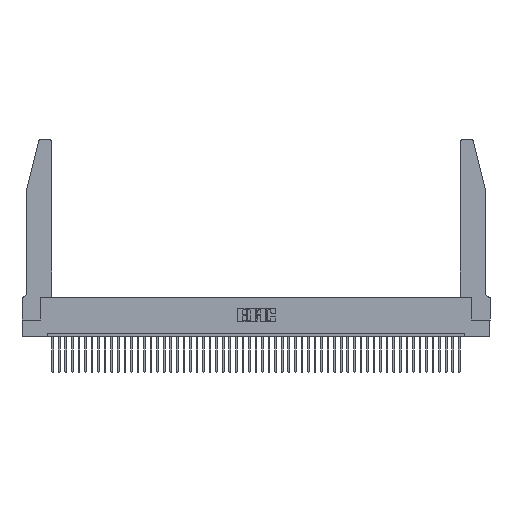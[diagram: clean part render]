
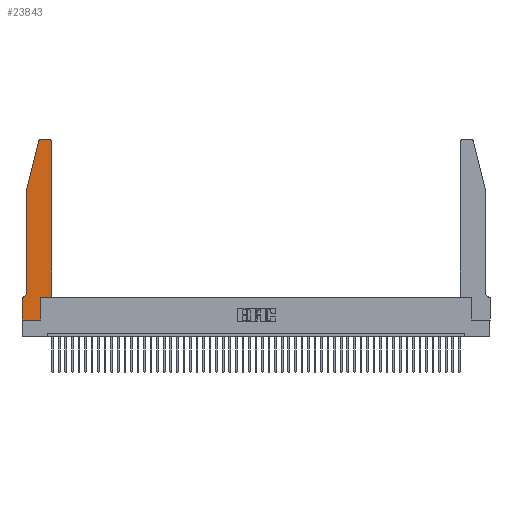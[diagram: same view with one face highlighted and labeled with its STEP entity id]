
A CAD part, top view. The second image highlights one B-rep face of the part: STEP entity #23843.
In plain terms, the highlighted planar face has unit normal (0, 0, 1).
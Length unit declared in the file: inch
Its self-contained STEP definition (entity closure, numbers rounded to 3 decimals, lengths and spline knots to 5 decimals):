
#1245 = DIRECTION ( 'NONE',  ( 1., 0., 0. ) ) ;
#1791 = LINE ( 'NONE', #37904, #36975 ) ;
#1830 = CARTESIAN_POINT ( 'NONE',  ( 0.4505, 0.35, 0.37 ) ) ;
#2072 = ORIENTED_EDGE ( 'NONE', *, *, #17591, .T. ) ;
#2438 = VERTEX_POINT ( 'NONE', #41297 ) ;
#2850 = AXIS2_PLACEMENT_3D ( 'NONE', #13372, #17579, #48704 ) ;
#2998 = EDGE_CURVE ( 'NONE', #13315, #28401, #1791, .T. ) ;
#3401 = LINE ( 'NONE', #48286, #9929 ) ;
#4139 = ORIENTED_EDGE ( 'NONE', *, *, #20110, .T. ) ;
#4287 = EDGE_CURVE ( 'NONE', #31102, #2438, #5827, .T. ) ;
#4763 = EDGE_CURVE ( 'NONE', #47648, #45885, #19547, .T. ) ;
#5475 = CARTESIAN_POINT ( 'NONE',  ( 0.2605, 2.75, 0.37 ) ) ;
#5827 = LINE ( 'NONE', #14766, #17216 ) ;
#6153 = LINE ( 'NONE', #5475, #27068 ) ;
#6427 = DIRECTION ( 'NONE',  ( 0., 1., 0. ) ) ;
#6703 = DIRECTION ( 'NONE',  ( 0., -1., 0. ) ) ;
#6869 = DIRECTION ( 'NONE',  ( 1., 0., 0. ) ) ;
#7040 = DIRECTION ( 'NONE',  ( 0., 0., 1. ) ) ;
#8311 = LINE ( 'NONE', #36016, #35166 ) ;
#8898 = DIRECTION ( 'NONE',  ( 0., 0., 1. ) ) ;
#9929 = VECTOR ( 'NONE', #6427, 39.37008 ) ;
#10194 = EDGE_CURVE ( 'NONE', #40480, #47648, #6153, .T. ) ;
#10562 = PLANE ( 'NONE',  #42308 ) ;
#11582 = AXIS2_PLACEMENT_3D ( 'NONE', #20313, #8898, #1245 ) ;
#11965 = VECTOR ( 'NONE', #31570, 39.37008 ) ;
#13315 = VERTEX_POINT ( 'NONE', #31732 ) ;
#13372 = CARTESIAN_POINT ( 'NONE',  ( 0.284, 2.72, 0.37 ) ) ;
#13621 = LINE ( 'NONE', #28148, #42801 ) ;
#13745 = CARTESIAN_POINT ( 'NONE',  ( 0.0755, 0.42, 0.37 ) ) ;
#14268 = CARTESIAN_POINT ( 'NONE',  ( 0.0055, 0.42, 0.37 ) ) ;
#14766 = CARTESIAN_POINT ( 'NONE',  ( 0., 0., 0.37 ) ) ;
#15083 = CARTESIAN_POINT ( 'NONE',  ( 0.4205, 2.75, 0.37 ) ) ;
#15116 = ORIENTED_EDGE ( 'NONE', *, *, #10194, .T. ) ;
#16860 = DIRECTION ( 'NONE',  ( 1., 0., 0. ) ) ;
#16972 = VERTEX_POINT ( 'NONE', #39715 ) ;
#17179 = ORIENTED_EDGE ( 'NONE', *, *, #45188, .T. ) ;
#17216 = VECTOR ( 'NONE', #26597, 39.37008 ) ;
#17579 = DIRECTION ( 'NONE',  ( 0., 0., 1. ) ) ;
#17591 = EDGE_CURVE ( 'NONE', #39319, #31102, #13621, .T. ) ;
#17788 = VECTOR ( 'NONE', #25382, 39.37008 ) ;
#18202 = FACE_OUTER_BOUND ( 'NONE', #48448, .T. ) ;
#19417 = ORIENTED_EDGE ( 'NONE', *, *, #29807, .T. ) ;
#19547 = CIRCLE ( 'NONE', #2850, 0.03 ) ;
#20110 = EDGE_CURVE ( 'NONE', #39949, #40480, #20575, .T. ) ;
#20198 = ORIENTED_EDGE ( 'NONE', *, *, #43814, .T. ) ;
#20313 = CARTESIAN_POINT ( 'NONE',  ( 0.4205, 2.72, 0.37 ) ) ;
#20343 = CARTESIAN_POINT ( 'NONE',  ( 0.284, 2.75, 0.37 ) ) ;
#20352 = LINE ( 'NONE', #48483, #25751 ) ;
#20575 = CIRCLE ( 'NONE', #11582, 0.03 ) ;
#21649 = DIRECTION ( 'NONE',  ( -1., 0., 0. ) ) ;
#22098 = CARTESIAN_POINT ( 'NONE',  ( 0., 0.35, 0.37 ) ) ;
#23573 = CARTESIAN_POINT ( 'NONE',  ( 0.4505, 0.35, 0.37 ) ) ;
#23843 = ADVANCED_FACE ( 'NONE', ( #18202 ), #10562, .T. ) ;
#24191 = DIRECTION ( 'NONE',  ( -1., 0., 0. ) ) ;
#25034 = ORIENTED_EDGE ( 'NONE', *, *, #39769, .T. ) ;
#25382 = DIRECTION ( 'NONE',  ( 0., 1., 0. ) ) ;
#25751 = VECTOR ( 'NONE', #30201, 39.37008 ) ;
#26597 = DIRECTION ( 'NONE',  ( 0., -1., 0. ) ) ;
#27068 = VECTOR ( 'NONE', #24191, 39.37008 ) ;
#27643 = ORIENTED_EDGE ( 'NONE', *, *, #32673, .T. ) ;
#28148 = CARTESIAN_POINT ( 'NONE',  ( 0.0755, 0.35, 0.37 ) ) ;
#28401 = VERTEX_POINT ( 'NONE', #13745 ) ;
#28522 = CARTESIAN_POINT ( 'NONE',  ( 0.4505, 0.35, 0.37 ) ) ;
#29807 = EDGE_CURVE ( 'NONE', #16972, #48147, #3401, .T. ) ;
#30201 = DIRECTION ( 'NONE',  ( -0.239, -0.971, 0. ) ) ;
#31102 = VERTEX_POINT ( 'NONE', #37093 ) ;
#31465 = CARTESIAN_POINT ( 'NONE',  ( 0.25487, 2.72718, 0.37 ) ) ;
#31570 = DIRECTION ( 'NONE',  ( 1., 0., 0. ) ) ;
#31732 = CARTESIAN_POINT ( 'NONE',  ( 0.0755, 2., 0.37 ) ) ;
#32673 = EDGE_CURVE ( 'NONE', #28401, #39319, #35885, .T. ) ;
#32940 = CARTESIAN_POINT ( 'NONE',  ( 0.2865, 0.35, 0.37 ) ) ;
#34564 = ORIENTED_EDGE ( 'NONE', *, *, #4763, .T. ) ;
#35166 = VECTOR ( 'NONE', #16860, 39.37008 ) ;
#35885 = CIRCLE ( 'NONE', #45480, 0.07 ) ;
#36016 = CARTESIAN_POINT ( 'NONE',  ( 0., 0., 0.37 ) ) ;
#36423 = ORIENTED_EDGE ( 'NONE', *, *, #4287, .T. ) ;
#36975 = VECTOR ( 'NONE', #6703, 39.37008 ) ;
#37093 = CARTESIAN_POINT ( 'NONE',  ( 0., 0.35, 0.37 ) ) ;
#37904 = CARTESIAN_POINT ( 'NONE',  ( 0.0755, 2., 0.37 ) ) ;
#39319 = VERTEX_POINT ( 'NONE', #41589 ) ;
#39715 = CARTESIAN_POINT ( 'NONE',  ( 0.2865, 0., 0.37 ) ) ;
#39769 = EDGE_CURVE ( 'NONE', #45885, #13315, #20352, .T. ) ;
#39949 = VERTEX_POINT ( 'NONE', #45279 ) ;
#40056 = LINE ( 'NONE', #23573, #11965 ) ;
#40480 = VERTEX_POINT ( 'NONE', #15083 ) ;
#40638 = DIRECTION ( 'NONE',  ( 0., 0., -1. ) ) ;
#41297 = CARTESIAN_POINT ( 'NONE',  ( 0., 0., 0.37 ) ) ;
#41589 = CARTESIAN_POINT ( 'NONE',  ( 0.0055, 0.35, 0.37 ) ) ;
#42308 = AXIS2_PLACEMENT_3D ( 'NONE', #22098, #7040, #6869 ) ;
#42801 = VECTOR ( 'NONE', #43317, 39.37008 ) ;
#43077 = EDGE_CURVE ( 'NONE', #48147, #45222, #40056, .T. ) ;
#43317 = DIRECTION ( 'NONE',  ( -1., 0., 0. ) ) ;
#43814 = EDGE_CURVE ( 'NONE', #2438, #16972, #8311, .T. ) ;
#44807 = ORIENTED_EDGE ( 'NONE', *, *, #2998, .T. ) ;
#45188 = EDGE_CURVE ( 'NONE', #45222, #39949, #49376, .T. ) ;
#45222 = VERTEX_POINT ( 'NONE', #28522 ) ;
#45279 = CARTESIAN_POINT ( 'NONE',  ( 0.4505, 2.72, 0.37 ) ) ;
#45367 = ORIENTED_EDGE ( 'NONE', *, *, #43077, .T. ) ;
#45480 = AXIS2_PLACEMENT_3D ( 'NONE', #14268, #40638, #21649 ) ;
#45885 = VERTEX_POINT ( 'NONE', #31465 ) ;
#47648 = VERTEX_POINT ( 'NONE', #20343 ) ;
#48147 = VERTEX_POINT ( 'NONE', #32940 ) ;
#48286 = CARTESIAN_POINT ( 'NONE',  ( 0.2865, 0.35, 0.37 ) ) ;
#48448 = EDGE_LOOP ( 'NONE', ( #15116, #34564, #25034, #44807, #27643, #2072, #36423, #20198, #19417, #45367, #17179, #4139 ) ) ;
#48483 = CARTESIAN_POINT ( 'NONE',  ( 0.0755, 2., 0.37 ) ) ;
#48704 = DIRECTION ( 'NONE',  ( 1., 0., 0. ) ) ;
#49376 = LINE ( 'NONE', #1830, #17788 ) ;
